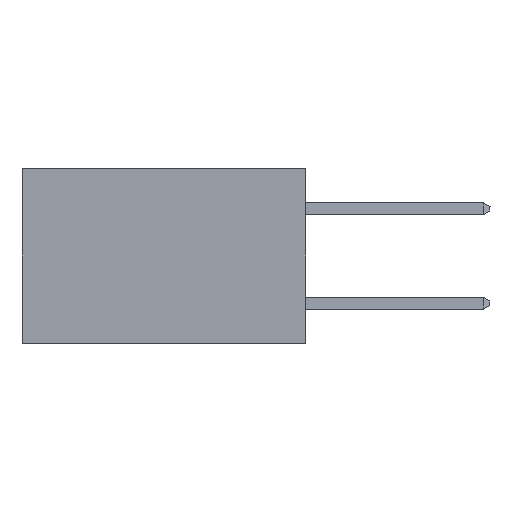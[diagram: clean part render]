
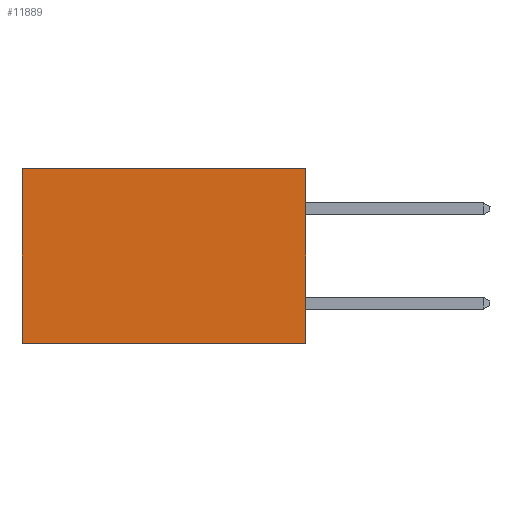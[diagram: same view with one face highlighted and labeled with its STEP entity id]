
A CAD part, left-side view. The second image highlights one B-rep face of the part: STEP entity #11889.
In plain terms, the highlighted planar face has unit normal (-1, 0, 0).
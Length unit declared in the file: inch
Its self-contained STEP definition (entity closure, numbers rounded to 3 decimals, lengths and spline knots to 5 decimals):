
#524 = EDGE_LOOP ( 'NONE', ( #23878, #6195, #17058, #20483 ) ) ;
#2305 = LINE ( 'NONE', #19538, #28222 ) ;
#2513 = EDGE_CURVE ( 'NONE', #3791, #20672, #19166, .T. ) ;
#2758 = VERTEX_POINT ( 'NONE', #25892 ) ;
#3791 = VERTEX_POINT ( 'NONE', #22174 ) ;
#4233 = VERTEX_POINT ( 'NONE', #23213 ) ;
#4814 = DIRECTION ( 'NONE',  ( 0., 0., -1. ) ) ;
#5806 = VECTOR ( 'NONE', #4814, 39.37008 ) ;
#6195 = ORIENTED_EDGE ( 'NONE', *, *, #14679, .F. ) ;
#7011 = DIRECTION ( 'NONE',  ( 0., 1., 0. ) ) ;
#8141 = PLANE ( 'NONE',  #15361 ) ;
#10617 = VECTOR ( 'NONE', #27524, 39.37008 ) ;
#11019 = FACE_OUTER_BOUND ( 'NONE', #524, .T. ) ;
#11889 = ADVANCED_FACE ( 'NONE', ( #11019 ), #8141, .F. ) ;
#12494 = CARTESIAN_POINT ( 'NONE',  ( 0.298, 0., -0.37 ) ) ;
#13180 = DIRECTION ( 'NONE',  ( 0., 0., -1. ) ) ;
#13337 = VECTOR ( 'NONE', #31801, 39.37008 ) ;
#14408 = CARTESIAN_POINT ( 'NONE',  ( 0.298, 0., 0. ) ) ;
#14679 = EDGE_CURVE ( 'NONE', #4233, #20672, #30531, .T. ) ;
#15361 = AXIS2_PLACEMENT_3D ( 'NONE', #25732, #28206, #13180 ) ;
#17058 = ORIENTED_EDGE ( 'NONE', *, *, #20811, .F. ) ;
#17234 = CARTESIAN_POINT ( 'NONE',  ( 0.298, 0.6, 0. ) ) ;
#19166 = LINE ( 'NONE', #17234, #5806 ) ;
#19538 = CARTESIAN_POINT ( 'NONE',  ( 0.298, 0., 0. ) ) ;
#20483 = ORIENTED_EDGE ( 'NONE', *, *, #26646, .T. ) ;
#20672 = VERTEX_POINT ( 'NONE', #23907 ) ;
#20811 = EDGE_CURVE ( 'NONE', #2758, #4233, #25937, .T. ) ;
#22174 = CARTESIAN_POINT ( 'NONE',  ( 0.298, 0.6, 0. ) ) ;
#23213 = CARTESIAN_POINT ( 'NONE',  ( 0.298, 0., -0.37 ) ) ;
#23878 = ORIENTED_EDGE ( 'NONE', *, *, #2513, .T. ) ;
#23907 = CARTESIAN_POINT ( 'NONE',  ( 0.298, 0.6, -0.37 ) ) ;
#25732 = CARTESIAN_POINT ( 'NONE',  ( 0.298, 0., 0. ) ) ;
#25892 = CARTESIAN_POINT ( 'NONE',  ( 0.298, 0., 0. ) ) ;
#25937 = LINE ( 'NONE', #14408, #13337 ) ;
#26646 = EDGE_CURVE ( 'NONE', #2758, #3791, #2305, .T. ) ;
#27524 = DIRECTION ( 'NONE',  ( 0., 1., 0. ) ) ;
#28206 = DIRECTION ( 'NONE',  ( 1., 0., 0. ) ) ;
#28222 = VECTOR ( 'NONE', #7011, 39.37008 ) ;
#30531 = LINE ( 'NONE', #12494, #10617 ) ;
#31801 = DIRECTION ( 'NONE',  ( 0., 0., -1. ) ) ;
